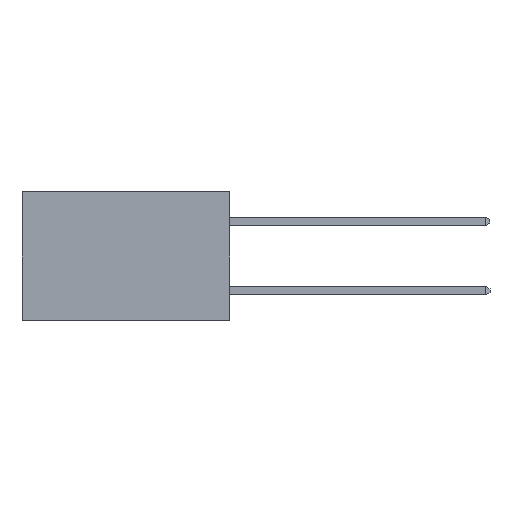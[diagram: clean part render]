
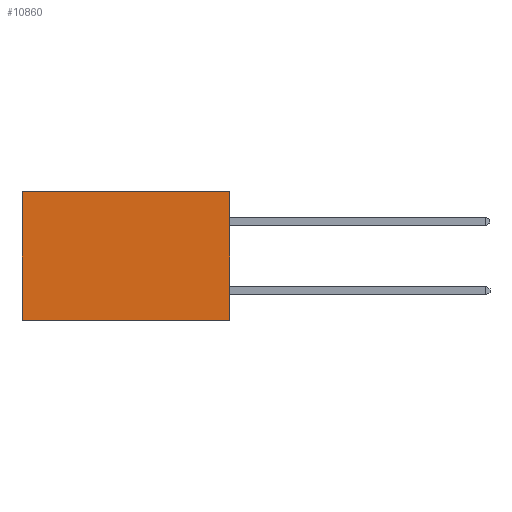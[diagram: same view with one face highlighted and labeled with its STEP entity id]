
A CAD part, left-side view. The second image highlights one B-rep face of the part: STEP entity #10860.
In plain terms, the highlighted planar face has unit normal (-1, 0, 0).
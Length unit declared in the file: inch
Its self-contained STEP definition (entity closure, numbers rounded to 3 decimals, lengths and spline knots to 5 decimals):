
#223 = VECTOR ( 'NONE', #8503, 39.37008 ) ;
#537 = EDGE_CURVE ( 'NONE', #876, #10218, #4716, .T. ) ;
#558 = DIRECTION ( 'NONE',  ( 0., 0., -1. ) ) ;
#876 = VERTEX_POINT ( 'NONE', #9959 ) ;
#1106 = EDGE_LOOP ( 'NONE', ( #2632, #6092, #7311, #2164 ) ) ;
#1209 = VERTEX_POINT ( 'NONE', #10515 ) ;
#1317 = CARTESIAN_POINT ( 'NONE',  ( 0.2615, 0., 0. ) ) ;
#2164 = ORIENTED_EDGE ( 'NONE', *, *, #9432, .T. ) ;
#2632 = ORIENTED_EDGE ( 'NONE', *, *, #537, .T. ) ;
#2840 = DIRECTION ( 'NONE',  ( 0., 0., -1. ) ) ;
#2933 = DIRECTION ( 'NONE',  ( 1., 0., 0. ) ) ;
#2963 = PLANE ( 'NONE',  #3359 ) ;
#3131 = CARTESIAN_POINT ( 'NONE',  ( 0.2615, 0., -0.37 ) ) ;
#3298 = DIRECTION ( 'NONE',  ( 0., 1., 0. ) ) ;
#3359 = AXIS2_PLACEMENT_3D ( 'NONE', #3131, #2933, #2840 ) ;
#3886 = VECTOR ( 'NONE', #9453, 39.37008 ) ;
#4555 = LINE ( 'NONE', #10237, #9089 ) ;
#4716 = LINE ( 'NONE', #9984, #9248 ) ;
#5339 = CARTESIAN_POINT ( 'NONE',  ( 0.2615, 0.6, -0.37 ) ) ;
#6092 = ORIENTED_EDGE ( 'NONE', *, *, #7455, .F. ) ;
#6295 = LINE ( 'NONE', #9575, #3886 ) ;
#7311 = ORIENTED_EDGE ( 'NONE', *, *, #7527, .F. ) ;
#7455 = EDGE_CURVE ( 'NONE', #1209, #10218, #11848, .T. ) ;
#7527 = EDGE_CURVE ( 'NONE', #9652, #1209, #6295, .T. ) ;
#8503 = DIRECTION ( 'NONE',  ( 0., 1., 0. ) ) ;
#8938 = CARTESIAN_POINT ( 'NONE',  ( 0.2615, 0., -0.37 ) ) ;
#9089 = VECTOR ( 'NONE', #3298, 39.37008 ) ;
#9248 = VECTOR ( 'NONE', #558, 39.37008 ) ;
#9432 = EDGE_CURVE ( 'NONE', #9652, #876, #4555, .T. ) ;
#9453 = DIRECTION ( 'NONE',  ( 0., 0., -1. ) ) ;
#9575 = CARTESIAN_POINT ( 'NONE',  ( 0.2615, 0., -0.37 ) ) ;
#9652 = VERTEX_POINT ( 'NONE', #1317 ) ;
#9959 = CARTESIAN_POINT ( 'NONE',  ( 0.2615, 0.6, 0. ) ) ;
#9984 = CARTESIAN_POINT ( 'NONE',  ( 0.2615, 0.6, -0.37 ) ) ;
#10218 = VERTEX_POINT ( 'NONE', #5339 ) ;
#10237 = CARTESIAN_POINT ( 'NONE',  ( 0.2615, 0., 0. ) ) ;
#10317 = FACE_OUTER_BOUND ( 'NONE', #1106, .T. ) ;
#10515 = CARTESIAN_POINT ( 'NONE',  ( 0.2615, 0., -0.37 ) ) ;
#10860 = ADVANCED_FACE ( 'NONE', ( #10317 ), #2963, .F. ) ;
#11848 = LINE ( 'NONE', #8938, #223 ) ;
